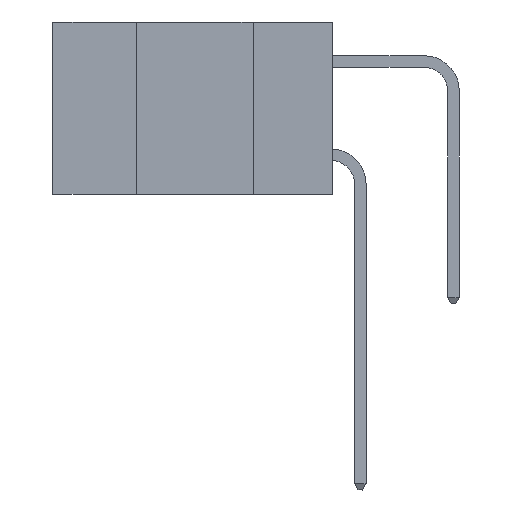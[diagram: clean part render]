
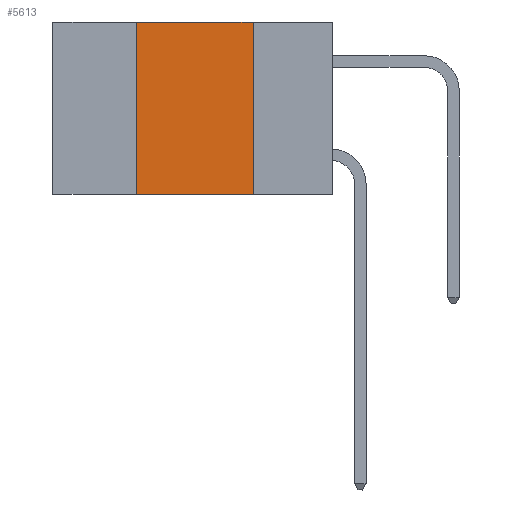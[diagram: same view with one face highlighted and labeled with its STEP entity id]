
A CAD part, left-side view. The second image highlights one B-rep face of the part: STEP entity #5613.
In plain terms, the highlighted planar face has unit normal (-1, 0, 0).
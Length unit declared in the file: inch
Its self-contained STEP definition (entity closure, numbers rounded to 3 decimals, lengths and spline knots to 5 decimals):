
#828 = CARTESIAN_POINT ( 'NONE',  ( 0., 0.17, -0.37 ) ) ;
#982 = VECTOR ( 'NONE', #11911, 39.37008 ) ;
#1010 = DIRECTION ( 'NONE',  ( 0., 0., 1. ) ) ;
#1144 = CARTESIAN_POINT ( 'NONE',  ( 0., 0.42, 0. ) ) ;
#1227 = VERTEX_POINT ( 'NONE', #11896 ) ;
#1642 = EDGE_CURVE ( 'NONE', #1227, #18415, #9360, .T. ) ;
#2115 = PLANE ( 'NONE',  #3317 ) ;
#2330 = CARTESIAN_POINT ( 'NONE',  ( 0., 0.6, 0. ) ) ;
#3317 = AXIS2_PLACEMENT_3D ( 'NONE', #2330, #8614, #8886 ) ;
#3408 = DIRECTION ( 'NONE',  ( 0., -1., 0. ) ) ;
#3453 = ORIENTED_EDGE ( 'NONE', *, *, #9937, .F. ) ;
#3659 = VECTOR ( 'NONE', #3408, 39.37008 ) ;
#5613 = ADVANCED_FACE ( 'NONE', ( #7483 ), #2115, .F. ) ;
#6834 = EDGE_CURVE ( 'NONE', #1227, #18161, #12598, .T. ) ;
#7069 = CARTESIAN_POINT ( 'NONE',  ( 0., 0.6, -0.37 ) ) ;
#7483 = FACE_OUTER_BOUND ( 'NONE', #8277, .T. ) ;
#7996 = ORIENTED_EDGE ( 'NONE', *, *, #1642, .T. ) ;
#8277 = EDGE_LOOP ( 'NONE', ( #3453, #16078, #15301, #7996 ) ) ;
#8614 = DIRECTION ( 'NONE',  ( 1., 0., 0. ) ) ;
#8886 = DIRECTION ( 'NONE',  ( 0., 0., -1. ) ) ;
#9360 = LINE ( 'NONE', #7069, #14779 ) ;
#9937 = EDGE_CURVE ( 'NONE', #10918, #18415, #16633, .T. ) ;
#10918 = VERTEX_POINT ( 'NONE', #18719 ) ;
#11442 = LINE ( 'NONE', #19323, #3659 ) ;
#11896 = CARTESIAN_POINT ( 'NONE',  ( 0., 0.42, -0.37 ) ) ;
#11911 = DIRECTION ( 'NONE',  ( 0., 0., -1. ) ) ;
#12598 = LINE ( 'NONE', #1144, #17747 ) ;
#12797 = CARTESIAN_POINT ( 'NONE',  ( 0., 0.42, 0. ) ) ;
#14779 = VECTOR ( 'NONE', #18191, 39.37008 ) ;
#15301 = ORIENTED_EDGE ( 'NONE', *, *, #6834, .F. ) ;
#16044 = EDGE_CURVE ( 'NONE', #18161, #10918, #11442, .T. ) ;
#16078 = ORIENTED_EDGE ( 'NONE', *, *, #16044, .F. ) ;
#16633 = LINE ( 'NONE', #17952, #982 ) ;
#17747 = VECTOR ( 'NONE', #1010, 39.37008 ) ;
#17952 = CARTESIAN_POINT ( 'NONE',  ( 0., 0.17, 0. ) ) ;
#18161 = VERTEX_POINT ( 'NONE', #12797 ) ;
#18191 = DIRECTION ( 'NONE',  ( 0., -1., 0. ) ) ;
#18415 = VERTEX_POINT ( 'NONE', #828 ) ;
#18719 = CARTESIAN_POINT ( 'NONE',  ( 0., 0.17, 0. ) ) ;
#19323 = CARTESIAN_POINT ( 'NONE',  ( 0., 0.6, 0. ) ) ;
